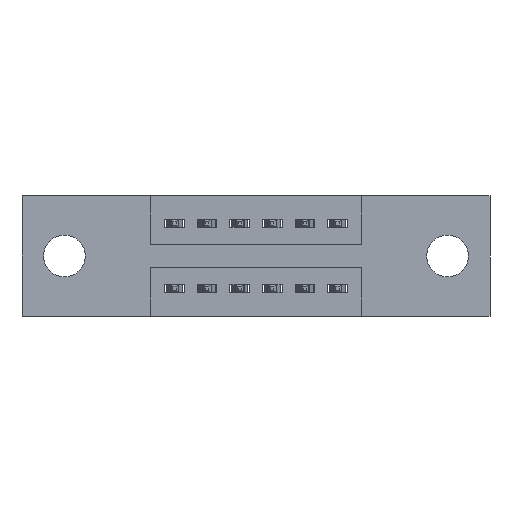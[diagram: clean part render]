
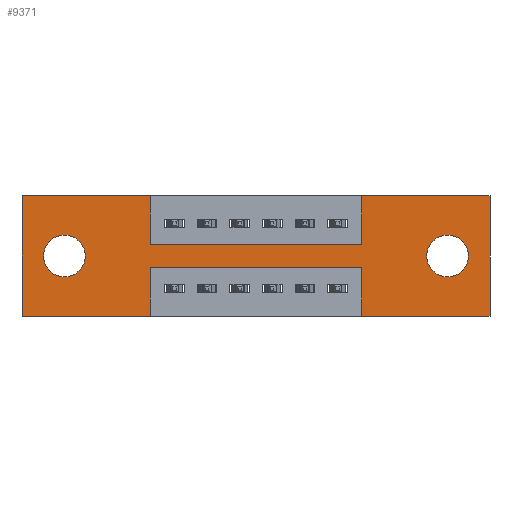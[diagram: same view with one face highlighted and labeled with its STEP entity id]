
A CAD part, front view. The second image highlights one B-rep face of the part: STEP entity #9371.
In plain terms, the highlighted planar face has unit normal (0, -1, 0).
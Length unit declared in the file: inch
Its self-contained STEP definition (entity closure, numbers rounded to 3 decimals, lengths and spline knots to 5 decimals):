
#30 = VERTEX_POINT ( 'NONE', #6152 ) ;
#188 = VERTEX_POINT ( 'NONE', #4761 ) ;
#319 = EDGE_CURVE ( 'NONE', #568, #1062, #4020, .T. ) ;
#357 = EDGE_LOOP ( 'NONE', ( #5002, #634, #6381, #4135, #2833, #3525, #1146, #1253, #4817, #6358, #4833, #6633 ) ) ;
#409 = FACE_BOUND ( 'NONE', #1898, .T. ) ;
#498 = CARTESIAN_POINT ( 'NONE',  ( 0.13, 0., -0.185 ) ) ;
#507 = LINE ( 'NONE', #2556, #5807 ) ;
#518 = EDGE_CURVE ( 'NONE', #4771, #3875, #7738, .T. ) ;
#523 = VERTEX_POINT ( 'NONE', #2324 ) ;
#568 = VERTEX_POINT ( 'NONE', #5252 ) ;
#629 = CARTESIAN_POINT ( 'NONE',  ( 0., 0., -0.37 ) ) ;
#634 = ORIENTED_EDGE ( 'NONE', *, *, #3624, .F. ) ;
#720 = AXIS2_PLACEMENT_3D ( 'NONE', #5346, #3119, #2425 ) ;
#831 = CIRCLE ( 'NONE', #5548, 0.064 ) ;
#857 = DIRECTION ( 'NONE',  ( 0., 0., -1. ) ) ;
#916 = ORIENTED_EDGE ( 'NONE', *, *, #319, .T. ) ;
#924 = CARTESIAN_POINT ( 'NONE',  ( 1.305, 0., -0.185 ) ) ;
#979 = CARTESIAN_POINT ( 'NONE',  ( 1.0425, 0., 0. ) ) ;
#1002 = CARTESIAN_POINT ( 'NONE',  ( 1.0425, 0., -0.37 ) ) ;
#1062 = VERTEX_POINT ( 'NONE', #5235 ) ;
#1086 = CARTESIAN_POINT ( 'NONE',  ( 0.3925, 0., -0.22 ) ) ;
#1146 = ORIENTED_EDGE ( 'NONE', *, *, #4208, .F. ) ;
#1207 = EDGE_CURVE ( 'NONE', #6297, #4771, #8590, .T. ) ;
#1241 = DIRECTION ( 'NONE',  ( 0., 1., 0. ) ) ;
#1253 = ORIENTED_EDGE ( 'NONE', *, *, #9114, .F. ) ;
#1445 = EDGE_CURVE ( 'NONE', #523, #3876, #3427, .T. ) ;
#1461 = LINE ( 'NONE', #6682, #4447 ) ;
#1511 = CARTESIAN_POINT ( 'NONE',  ( 1.435, 0., 0. ) ) ;
#1557 = EDGE_LOOP ( 'NONE', ( #9539, #8761 ) ) ;
#1600 = CARTESIAN_POINT ( 'NONE',  ( 0., 0., -0.37 ) ) ;
#1655 = FACE_BOUND ( 'NONE', #1557, .T. ) ;
#1898 = EDGE_LOOP ( 'NONE', ( #7807, #916 ) ) ;
#1988 = DIRECTION ( 'NONE',  ( 0., 0., -1. ) ) ;
#2026 = AXIS2_PLACEMENT_3D ( 'NONE', #924, #6076, #2405 ) ;
#2050 = VERTEX_POINT ( 'NONE', #1511 ) ;
#2075 = CARTESIAN_POINT ( 'NONE',  ( 1.435, 0., 0. ) ) ;
#2168 = VECTOR ( 'NONE', #4691, 39.37008 ) ;
#2302 = CARTESIAN_POINT ( 'NONE',  ( 0., 0., 0. ) ) ;
#2324 = CARTESIAN_POINT ( 'NONE',  ( 1.305, 0., -0.121 ) ) ;
#2373 = VECTOR ( 'NONE', #9310, 39.37008 ) ;
#2405 = DIRECTION ( 'NONE',  ( 0., 0., -1. ) ) ;
#2425 = DIRECTION ( 'NONE',  ( 0., 0., -1. ) ) ;
#2506 = DIRECTION ( 'NONE',  ( 0., 0., 1. ) ) ;
#2544 = DIRECTION ( 'NONE',  ( 0., -1., 0. ) ) ;
#2556 = CARTESIAN_POINT ( 'NONE',  ( 0.3925, 0., -0.15 ) ) ;
#2676 = CARTESIAN_POINT ( 'NONE',  ( 0., 0., 0. ) ) ;
#2735 = VERTEX_POINT ( 'NONE', #3405 ) ;
#2833 = ORIENTED_EDGE ( 'NONE', *, *, #5393, .F. ) ;
#2879 = CARTESIAN_POINT ( 'NONE',  ( 0.3925, 0., -0.37 ) ) ;
#2883 = DIRECTION ( 'NONE',  ( 0., 0., -1. ) ) ;
#2918 = LINE ( 'NONE', #6042, #6989 ) ;
#3010 = EDGE_CURVE ( 'NONE', #30, #5571, #6785, .T. ) ;
#3018 = DIRECTION ( 'NONE',  ( -1., 0., 0. ) ) ;
#3045 = EDGE_CURVE ( 'NONE', #6517, #2050, #7858, .T. ) ;
#3119 = DIRECTION ( 'NONE',  ( 0., 1., 0. ) ) ;
#3317 = DIRECTION ( 'NONE',  ( 1., 0., 0. ) ) ;
#3405 = CARTESIAN_POINT ( 'NONE',  ( 1.0425, 0., -0.15 ) ) ;
#3427 = CIRCLE ( 'NONE', #720, 0.064 ) ;
#3496 = CARTESIAN_POINT ( 'NONE',  ( 0.3925, 0., -0.15 ) ) ;
#3525 = ORIENTED_EDGE ( 'NONE', *, *, #3045, .F. ) ;
#3624 = EDGE_CURVE ( 'NONE', #188, #6297, #1461, .T. ) ;
#3843 = VECTOR ( 'NONE', #857, 39.37008 ) ;
#3875 = VERTEX_POINT ( 'NONE', #629 ) ;
#3876 = VERTEX_POINT ( 'NONE', #5758 ) ;
#3901 = DIRECTION ( 'NONE',  ( 0., 0., 1. ) ) ;
#3993 = CARTESIAN_POINT ( 'NONE',  ( 1.0425, 0., -0.37 ) ) ;
#4020 = CIRCLE ( 'NONE', #4279, 0.064 ) ;
#4071 = EDGE_CURVE ( 'NONE', #3876, #523, #7829, .T. ) ;
#4135 = ORIENTED_EDGE ( 'NONE', *, *, #3010, .F. ) ;
#4208 = EDGE_CURVE ( 'NONE', #2735, #6517, #8994, .T. ) ;
#4221 = EDGE_CURVE ( 'NONE', #3875, #7700, #5719, .T. ) ;
#4279 = AXIS2_PLACEMENT_3D ( 'NONE', #498, #1241, #7906 ) ;
#4447 = VECTOR ( 'NONE', #3018, 39.37008 ) ;
#4477 = CARTESIAN_POINT ( 'NONE',  ( 1.0425, 0., 0. ) ) ;
#4675 = DIRECTION ( 'NONE',  ( 0., 0., 1. ) ) ;
#4691 = DIRECTION ( 'NONE',  ( 1., 0., 0. ) ) ;
#4761 = CARTESIAN_POINT ( 'NONE',  ( 1.0425, 0., -0.22 ) ) ;
#4771 = VERTEX_POINT ( 'NONE', #5625 ) ;
#4817 = ORIENTED_EDGE ( 'NONE', *, *, #4963, .F. ) ;
#4833 = ORIENTED_EDGE ( 'NONE', *, *, #4221, .F. ) ;
#4963 = EDGE_CURVE ( 'NONE', #7205, #8928, #7923, .T. ) ;
#5002 = ORIENTED_EDGE ( 'NONE', *, *, #1207, .F. ) ;
#5059 = VECTOR ( 'NONE', #5937, 39.37008 ) ;
#5115 = FACE_OUTER_BOUND ( 'NONE', #357, .T. ) ;
#5180 = CARTESIAN_POINT ( 'NONE',  ( 0.3925, 0., 0. ) ) ;
#5235 = CARTESIAN_POINT ( 'NONE',  ( 0.13, 0., -0.121 ) ) ;
#5252 = CARTESIAN_POINT ( 'NONE',  ( 0.13, 0., -0.249 ) ) ;
#5342 = DIRECTION ( 'NONE',  ( -1., 0., 0. ) ) ;
#5346 = CARTESIAN_POINT ( 'NONE',  ( 1.305, 0., -0.185 ) ) ;
#5393 = EDGE_CURVE ( 'NONE', #2050, #30, #8623, .T. ) ;
#5548 = AXIS2_PLACEMENT_3D ( 'NONE', #7679, #6231, #4675 ) ;
#5571 = VERTEX_POINT ( 'NONE', #3993 ) ;
#5597 = CARTESIAN_POINT ( 'NONE',  ( 0.3925, 0., 0. ) ) ;
#5625 = CARTESIAN_POINT ( 'NONE',  ( 0.3925, 0., -0.37 ) ) ;
#5694 = AXIS2_PLACEMENT_3D ( 'NONE', #9393, #2544, #1988 ) ;
#5696 = PLANE ( 'NONE',  #5694 ) ;
#5719 = LINE ( 'NONE', #2676, #6290 ) ;
#5758 = CARTESIAN_POINT ( 'NONE',  ( 1.305, 0., -0.249 ) ) ;
#5767 = VECTOR ( 'NONE', #8089, 39.37008 ) ;
#5807 = VECTOR ( 'NONE', #3317, 39.37008 ) ;
#5937 = DIRECTION ( 'NONE',  ( -1., 0., 0. ) ) ;
#6042 = CARTESIAN_POINT ( 'NONE',  ( 0., 0., 0. ) ) ;
#6076 = DIRECTION ( 'NONE',  ( 0., 1., 0. ) ) ;
#6152 = CARTESIAN_POINT ( 'NONE',  ( 1.435, 0., -0.37 ) ) ;
#6210 = EDGE_CURVE ( 'NONE', #1062, #568, #831, .T. ) ;
#6231 = DIRECTION ( 'NONE',  ( 0., 1., 0. ) ) ;
#6290 = VECTOR ( 'NONE', #3901, 39.37008 ) ;
#6297 = VERTEX_POINT ( 'NONE', #1086 ) ;
#6358 = ORIENTED_EDGE ( 'NONE', *, *, #8082, .F. ) ;
#6381 = ORIENTED_EDGE ( 'NONE', *, *, #8404, .F. ) ;
#6517 = VERTEX_POINT ( 'NONE', #4477 ) ;
#6629 = LINE ( 'NONE', #1002, #7817 ) ;
#6633 = ORIENTED_EDGE ( 'NONE', *, *, #518, .F. ) ;
#6682 = CARTESIAN_POINT ( 'NONE',  ( 0.3925, 0., -0.22 ) ) ;
#6785 = LINE ( 'NONE', #1600, #5059 ) ;
#6989 = VECTOR ( 'NONE', #9024, 39.37008 ) ;
#7205 = VERTEX_POINT ( 'NONE', #5597 ) ;
#7387 = CARTESIAN_POINT ( 'NONE',  ( 0., 0., 0. ) ) ;
#7570 = CARTESIAN_POINT ( 'NONE',  ( 0., 0., -0.37 ) ) ;
#7679 = CARTESIAN_POINT ( 'NONE',  ( 0.13, 0., -0.185 ) ) ;
#7700 = VERTEX_POINT ( 'NONE', #2302 ) ;
#7738 = LINE ( 'NONE', #7570, #8910 ) ;
#7807 = ORIENTED_EDGE ( 'NONE', *, *, #6210, .T. ) ;
#7817 = VECTOR ( 'NONE', #2506, 39.37008 ) ;
#7829 = CIRCLE ( 'NONE', #2026, 0.064 ) ;
#7858 = LINE ( 'NONE', #7387, #2168 ) ;
#7906 = DIRECTION ( 'NONE',  ( 0., 0., 1. ) ) ;
#7923 = LINE ( 'NONE', #5180, #3843 ) ;
#8031 = VECTOR ( 'NONE', #2883, 39.37008 ) ;
#8082 = EDGE_CURVE ( 'NONE', #7700, #7205, #2918, .T. ) ;
#8089 = DIRECTION ( 'NONE',  ( 0., 0., -1. ) ) ;
#8404 = EDGE_CURVE ( 'NONE', #5571, #188, #6629, .T. ) ;
#8590 = LINE ( 'NONE', #2879, #5767 ) ;
#8623 = LINE ( 'NONE', #2075, #8031 ) ;
#8761 = ORIENTED_EDGE ( 'NONE', *, *, #4071, .T. ) ;
#8910 = VECTOR ( 'NONE', #5342, 39.37008 ) ;
#8928 = VERTEX_POINT ( 'NONE', #3496 ) ;
#8994 = LINE ( 'NONE', #979, #2373 ) ;
#9024 = DIRECTION ( 'NONE',  ( 1., 0., 0. ) ) ;
#9114 = EDGE_CURVE ( 'NONE', #8928, #2735, #507, .T. ) ;
#9310 = DIRECTION ( 'NONE',  ( 0., 0., 1. ) ) ;
#9371 = ADVANCED_FACE ( 'NONE', ( #1655, #409, #5115 ), #5696, .T. ) ;
#9393 = CARTESIAN_POINT ( 'NONE',  ( 0., 0., -0.37 ) ) ;
#9539 = ORIENTED_EDGE ( 'NONE', *, *, #1445, .T. ) ;
